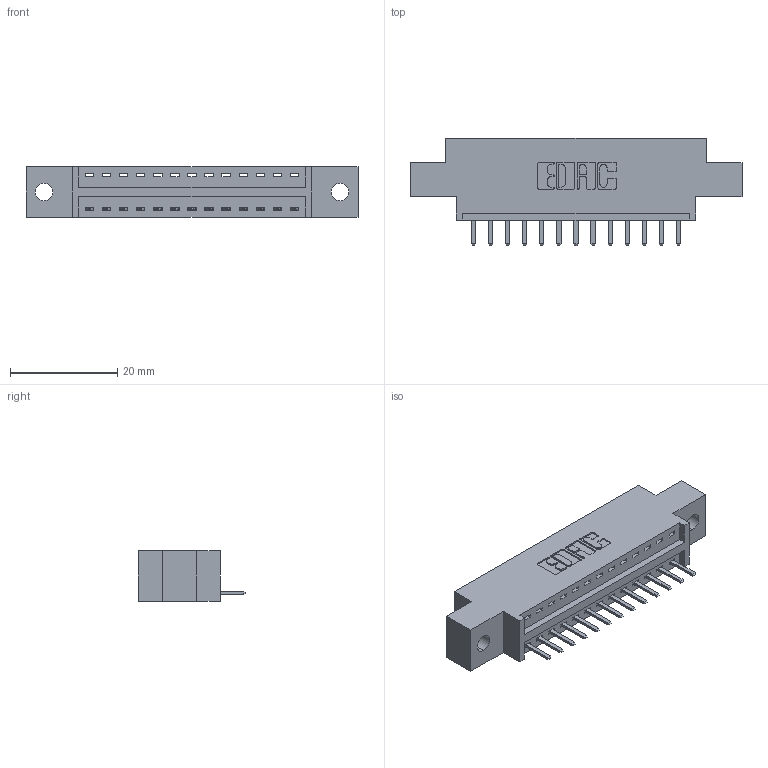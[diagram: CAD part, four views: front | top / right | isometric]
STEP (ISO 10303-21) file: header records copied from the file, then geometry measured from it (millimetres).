
FILE_DESCRIPTION (( 'STEP AP203' ), '1' );
FILE_NAME ('396-013-520-602.STEP', '2019-10-26T15:52:38', ( '' ), ( '' ), 'SwSTEP 2.0', 'SolidWorks 2016', '' );
FILE_SCHEMA (( 'CONFIG_CONTROL_DESIGN' ));
Length unit declared in the file: inch
Products named in the file (3): 346 Part_0.170 Offset - 0.128 Dia; 396-013-520-602; 345-292-001_345-293-120
Assembly tree (14 placements, depth 2):
  396-013-520-602
    346 Part_0.170 Offset - 0.128 Dia
    345-292-001_345-293-120  x13
Bounding box: 61.85 x 20.02 x 9.4 mm (x, y, z)
Volume: 5491.8 mm3; surface area: 6315.4 mm2
Topology: 14 solids, 14 shells, 932 faces, 2733 edges, 1786 vertices
Faces by surface type: plane 626, cylinder 306
Entity records: 12221 total; most frequent: CARTESIAN_POINT 2123, ORIENTED_EDGE 2058, DIRECTION 1895, EDGE_CURVE 1029, VECTOR 841, LINE 841, VERTEX_POINT 682, AXIS2_PLACEMENT_3D 527
